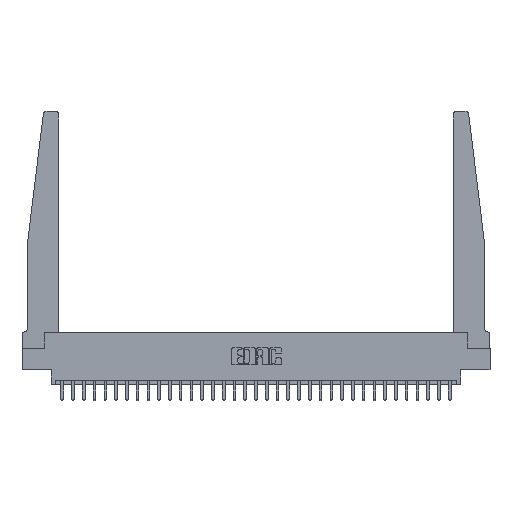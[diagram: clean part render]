
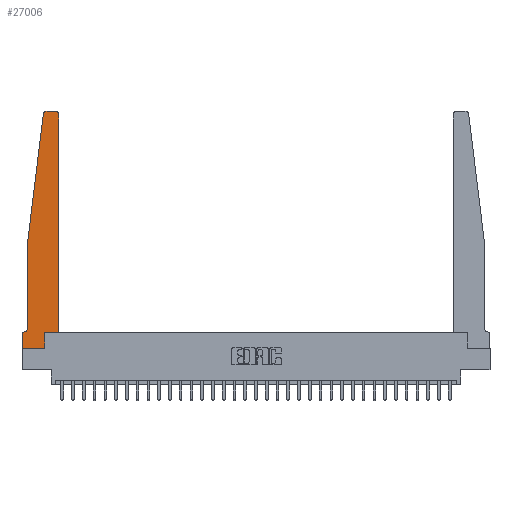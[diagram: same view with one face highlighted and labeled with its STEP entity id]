
A CAD part, top view. The second image highlights one B-rep face of the part: STEP entity #27006.
In plain terms, the highlighted planar face has unit normal (0, 0, 1).
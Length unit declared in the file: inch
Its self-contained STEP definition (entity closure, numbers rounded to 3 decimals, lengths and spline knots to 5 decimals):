
#123 = CARTESIAN_POINT ( 'NONE',  ( 0.2605, 0., 0.37 ) ) ;
#1237 = CARTESIAN_POINT ( 'NONE',  ( 0.015, 0.2375, 0.37 ) ) ;
#1310 = EDGE_CURVE ( 'NONE', #19576, #14174, #3849, .T. ) ;
#1964 = LINE ( 'NONE', #18980, #25775 ) ;
#3484 = VERTEX_POINT ( 'NONE', #26952 ) ;
#3537 = DIRECTION ( 'NONE',  ( -1., 0., 0. ) ) ;
#3785 = LINE ( 'NONE', #9583, #26162 ) ;
#3849 = LINE ( 'NONE', #22942, #29839 ) ;
#4267 = VERTEX_POINT ( 'NONE', #15724 ) ;
#4672 = CIRCLE ( 'NONE', #8210, 0.05 ) ;
#4923 = DIRECTION ( 'NONE',  ( 0., 0., 1. ) ) ;
#5487 = DIRECTION ( 'NONE',  ( -1., 0., 0. ) ) ;
#5552 = ORIENTED_EDGE ( 'NONE', *, *, #19735, .T. ) ;
#6074 = CARTESIAN_POINT ( 'NONE',  ( 0.2605, 0.18, 0.37 ) ) ;
#6553 = AXIS2_PLACEMENT_3D ( 'NONE', #18772, #4923, #21069 ) ;
#6990 = LINE ( 'NONE', #28600, #18550 ) ;
#7151 = CARTESIAN_POINT ( 'NONE',  ( 0., 0.1875, 0.37 ) ) ;
#7392 = VERTEX_POINT ( 'NONE', #22728 ) ;
#7465 = LINE ( 'NONE', #14785, #8214 ) ;
#7681 = DIRECTION ( 'NONE',  ( -0.122, -0.992, 0. ) ) ;
#8210 = AXIS2_PLACEMENT_3D ( 'NONE', #1237, #17397, #3537 ) ;
#8214 = VECTOR ( 'NONE', #26165, 39.37008 ) ;
#8493 = EDGE_CURVE ( 'NONE', #11783, #21546, #13311, .T. ) ;
#8569 = VECTOR ( 'NONE', #29180, 39.37008 ) ;
#9109 = ORIENTED_EDGE ( 'NONE', *, *, #9456, .T. ) ;
#9294 = ORIENTED_EDGE ( 'NONE', *, *, #18178, .T. ) ;
#9456 = EDGE_CURVE ( 'NONE', #21546, #14967, #1964, .T. ) ;
#9491 = DIRECTION ( 'NONE',  ( 0., 0., 1. ) ) ;
#9551 = EDGE_CURVE ( 'NONE', #27967, #7392, #19645, .T. ) ;
#9583 = CARTESIAN_POINT ( 'NONE',  ( 0.25, 2.75, 0.37 ) ) ;
#9808 = CARTESIAN_POINT ( 'NONE',  ( 0.27653, 2.72, 0.37 ) ) ;
#9889 = CARTESIAN_POINT ( 'NONE',  ( 0.425, 0.18, 0.37 ) ) ;
#9934 = ORIENTED_EDGE ( 'NONE', *, *, #1310, .T. ) ;
#10384 = CARTESIAN_POINT ( 'NONE',  ( 0., 0., 0.37 ) ) ;
#10450 = EDGE_CURVE ( 'NONE', #24696, #11783, #6990, .T. ) ;
#11186 = AXIS2_PLACEMENT_3D ( 'NONE', #9808, #25915, #12114 ) ;
#11457 = DIRECTION ( 'NONE',  ( 0., -1., 0. ) ) ;
#11698 = CARTESIAN_POINT ( 'NONE',  ( 0., 0., 0.37 ) ) ;
#11783 = VERTEX_POINT ( 'NONE', #12826 ) ;
#12114 = DIRECTION ( 'NONE',  ( 1., 0., 0. ) ) ;
#12528 = CARTESIAN_POINT ( 'NONE',  ( 0.425, 2.72, 0.37 ) ) ;
#12579 = VECTOR ( 'NONE', #28318, 39.37008 ) ;
#12752 = FACE_OUTER_BOUND ( 'NONE', #22214, .T. ) ;
#12826 = CARTESIAN_POINT ( 'NONE',  ( 0., 0.1875, 0.37 ) ) ;
#13180 = LINE ( 'NONE', #6074, #8569 ) ;
#13311 = LINE ( 'NONE', #10384, #14031 ) ;
#13767 = VECTOR ( 'NONE', #7681, 39.37008 ) ;
#14031 = VECTOR ( 'NONE', #24178, 39.37008 ) ;
#14174 = VERTEX_POINT ( 'NONE', #29399 ) ;
#14488 = LINE ( 'NONE', #19284, #13767 ) ;
#14558 = ORIENTED_EDGE ( 'NONE', *, *, #9551, .T. ) ;
#14785 = CARTESIAN_POINT ( 'NONE',  ( 0.425, 0.18, 0.37 ) ) ;
#14967 = VERTEX_POINT ( 'NONE', #123 ) ;
#15283 = CARTESIAN_POINT ( 'NONE',  ( 0.015, 0.1875, 0.37 ) ) ;
#15437 = VERTEX_POINT ( 'NONE', #24702 ) ;
#15724 = CARTESIAN_POINT ( 'NONE',  ( 0.425, 0.18, 0.37 ) ) ;
#15903 = ORIENTED_EDGE ( 'NONE', *, *, #15928, .T. ) ;
#15928 = EDGE_CURVE ( 'NONE', #14967, #3484, #13180, .T. ) ;
#16102 = AXIS2_PLACEMENT_3D ( 'NONE', #7151, #9491, #25612 ) ;
#17114 = ORIENTED_EDGE ( 'NONE', *, *, #28165, .T. ) ;
#17397 = DIRECTION ( 'NONE',  ( 0., 0., -1. ) ) ;
#18161 = CARTESIAN_POINT ( 'NONE',  ( 0.065, 1.25, 0.37 ) ) ;
#18178 = EDGE_CURVE ( 'NONE', #14174, #24696, #4672, .T. ) ;
#18550 = VECTOR ( 'NONE', #5487, 39.37008 ) ;
#18772 = CARTESIAN_POINT ( 'NONE',  ( 0.395, 2.72, 0.37 ) ) ;
#18980 = CARTESIAN_POINT ( 'NONE',  ( 0., 0., 0.37 ) ) ;
#19245 = VERTEX_POINT ( 'NONE', #12528 ) ;
#19284 = CARTESIAN_POINT ( 'NONE',  ( 0.065, 1.25, 0.37 ) ) ;
#19576 = VERTEX_POINT ( 'NONE', #18161 ) ;
#19645 = CIRCLE ( 'NONE', #11186, 0.03 ) ;
#19735 = EDGE_CURVE ( 'NONE', #4267, #19245, #20132, .T. ) ;
#20132 = LINE ( 'NONE', #9889, #12579 ) ;
#20376 = ORIENTED_EDGE ( 'NONE', *, *, #25140, .T. ) ;
#20838 = ORIENTED_EDGE ( 'NONE', *, *, #10450, .T. ) ;
#20993 = CARTESIAN_POINT ( 'NONE',  ( 0.27653, 2.75, 0.37 ) ) ;
#21069 = DIRECTION ( 'NONE',  ( 1., 0., 0. ) ) ;
#21279 = DIRECTION ( 'NONE',  ( 1., 0., 0. ) ) ;
#21546 = VERTEX_POINT ( 'NONE', #11698 ) ;
#21593 = EDGE_CURVE ( 'NONE', #15437, #27967, #3785, .T. ) ;
#22214 = EDGE_LOOP ( 'NONE', ( #24521, #14558, #17114, #9934, #9294, #20838, #24830, #9109, #15903, #27233, #5552, #20376 ) ) ;
#22728 = CARTESIAN_POINT ( 'NONE',  ( 0.24675, 2.72367, 0.37 ) ) ;
#22942 = CARTESIAN_POINT ( 'NONE',  ( 0.065, 1.25, 0.37 ) ) ;
#23287 = PLANE ( 'NONE',  #16102 ) ;
#23371 = DIRECTION ( 'NONE',  ( -1., 0., 0. ) ) ;
#24178 = DIRECTION ( 'NONE',  ( 0., -1., 0. ) ) ;
#24403 = CIRCLE ( 'NONE', #6553, 0.03 ) ;
#24521 = ORIENTED_EDGE ( 'NONE', *, *, #21593, .T. ) ;
#24556 = EDGE_CURVE ( 'NONE', #3484, #4267, #7465, .T. ) ;
#24696 = VERTEX_POINT ( 'NONE', #15283 ) ;
#24702 = CARTESIAN_POINT ( 'NONE',  ( 0.395, 2.75, 0.37 ) ) ;
#24830 = ORIENTED_EDGE ( 'NONE', *, *, #8493, .T. ) ;
#25140 = EDGE_CURVE ( 'NONE', #19245, #15437, #24403, .T. ) ;
#25612 = DIRECTION ( 'NONE',  ( 1., 0., 0. ) ) ;
#25775 = VECTOR ( 'NONE', #21279, 39.37008 ) ;
#25915 = DIRECTION ( 'NONE',  ( 0., 0., 1. ) ) ;
#26162 = VECTOR ( 'NONE', #23371, 39.37008 ) ;
#26165 = DIRECTION ( 'NONE',  ( 1., 0., 0. ) ) ;
#26952 = CARTESIAN_POINT ( 'NONE',  ( 0.2605, 0.18, 0.37 ) ) ;
#27006 = ADVANCED_FACE ( 'NONE', ( #12752 ), #23287, .T. ) ;
#27233 = ORIENTED_EDGE ( 'NONE', *, *, #24556, .T. ) ;
#27967 = VERTEX_POINT ( 'NONE', #20993 ) ;
#28165 = EDGE_CURVE ( 'NONE', #7392, #19576, #14488, .T. ) ;
#28318 = DIRECTION ( 'NONE',  ( 0., 1., 0. ) ) ;
#28600 = CARTESIAN_POINT ( 'NONE',  ( 0.065, 0.1875, 0.37 ) ) ;
#29180 = DIRECTION ( 'NONE',  ( 0., 1., 0. ) ) ;
#29399 = CARTESIAN_POINT ( 'NONE',  ( 0.065, 0.2375, 0.37 ) ) ;
#29839 = VECTOR ( 'NONE', #11457, 39.37008 ) ;
